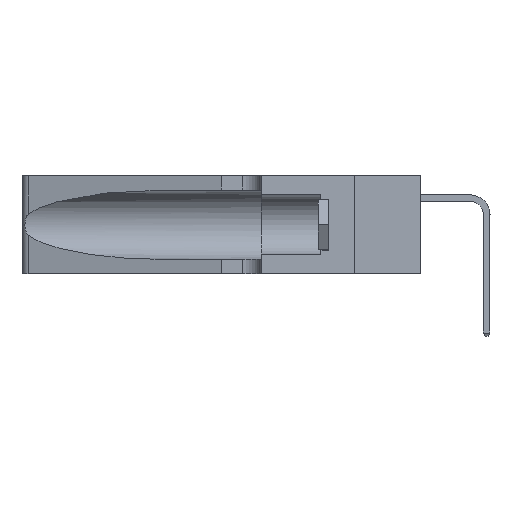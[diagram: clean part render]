
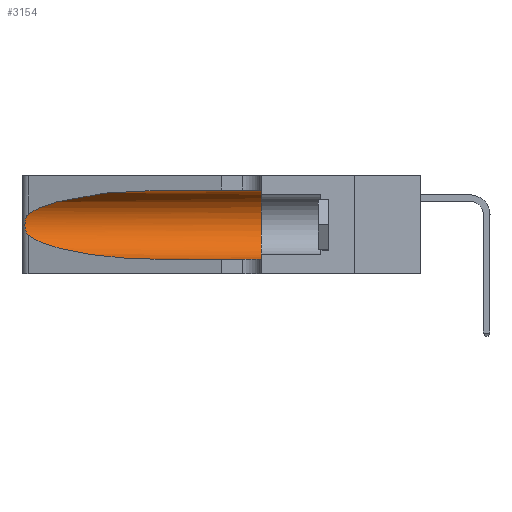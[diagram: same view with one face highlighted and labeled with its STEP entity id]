
A CAD part, left-side view. The second image highlights one B-rep face of the part: STEP entity #3154.
In plain terms, the highlighted cylindrical face has radius 3.308 mm (diameter 6.617 mm), a partial arc.
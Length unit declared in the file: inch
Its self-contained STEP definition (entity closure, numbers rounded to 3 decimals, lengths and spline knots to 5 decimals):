
#513 = CARTESIAN_POINT ( 'NONE',  ( 0.2373, 1.15595, 0.28018 ) ) ;
#948 = CARTESIAN_POINT ( 'NONE',  ( 0.25856, 1.23593, 0.16098 ) ) ;
#1229 = CARTESIAN_POINT ( 'NONE',  ( 0.1305, 1.61858, 0.31525 ) ) ;
#1253 = ORIENTED_EDGE ( 'NONE', *, *, #3445, .T. ) ;
#2383 = CARTESIAN_POINT ( 'NONE',  ( 0.25487, 1.22718, 0.22369 ) ) ;
#2447 = CARTESIAN_POINT ( 'NONE',  ( 0.25639, 1.23186, 0.15144 ) ) ;
#3079 = CYLINDRICAL_SURFACE ( 'NONE', #17905, 0.13025 ) ;
#3154 = ADVANCED_FACE ( 'NONE', ( #14807 ), #3079, .F. ) ;
#3445 = EDGE_CURVE ( 'NONE', #12646, #9688, #5342, .T. ) ;
#3483 = CARTESIAN_POINT ( 'NONE',  ( 0.1305, 1.61858, 0.185 ) ) ;
#3907 = CARTESIAN_POINT ( 'NONE',  ( 0.25487, 1.22718, 0.14631 ) ) ;
#3959 = ORIENTED_EDGE ( 'NONE', *, *, #9111, .T. ) ;
#4070 = VECTOR ( 'NONE', #13001, 39.37008 ) ;
#4878 = CARTESIAN_POINT ( 'NONE',  ( 0.1305, 0.35, 0.05475 ) ) ;
#5135 = CARTESIAN_POINT ( 'NONE',  ( 0.1305, 0.72297, 0.05475 ) ) ;
#5319 = CARTESIAN_POINT ( 'NONE',  ( 0.25639, 1.23184, 0.21858 ) ) ;
#5342 = LINE ( 'NONE', #17553, #16624 ) ;
#5837 = VERTEX_POINT ( 'NONE', #18272 ) ;
#5860 = DIRECTION ( 'NONE',  ( 0., -1., 0. ) ) ;
#6227 = ORIENTED_EDGE ( 'NONE', *, *, #8762, .F. ) ;
#6828 = CARTESIAN_POINT ( 'NONE',  ( 0.25854, 1.2359, 0.20912 ) ) ;
#7110 = DIRECTION ( 'NONE',  ( 0., 1., 0. ) ) ;
#7113 = ORIENTED_EDGE ( 'NONE', *, *, #17743, .F. ) ;
#7295 = EDGE_LOOP ( 'NONE', ( #3959, #17143, #15852, #1253, #6227, #7113 ) ) ;
#7996 = LINE ( 'NONE', #1229, #4070 ) ;
#8301 = CARTESIAN_POINT ( 'NONE',  ( 0.26075, 1.23896, 0.19203 ) ) ;
#8713 = CIRCLE ( 'NONE', #17393, 0.13025 ) ;
#8762 = EDGE_CURVE ( 'NONE', #18792, #9688, #8713, .T. ) ;
#9111 = EDGE_CURVE ( 'NONE', #12987, #5837, #9203, .T. ) ;
#9203 =( BOUNDED_CURVE ( )  B_SPLINE_CURVE ( 3, ( #15119, #15186, #513, #10826 ),
 .UNSPECIFIED., .F., .F. ) 
 B_SPLINE_CURVE_WITH_KNOTS ( ( 4, 4 ),
 ( 1.5708, 2.84003 ),
 .UNSPECIFIED. ) 
 CURVE ( )  GEOMETRIC_REPRESENTATION_ITEM ( )  RATIONAL_B_SPLINE_CURVE ( ( 1., 0.87, 0.87, 1. ) ) 
 REPRESENTATION_ITEM ( '' )  );
#9494 = CARTESIAN_POINT ( 'NONE',  ( 0.2373, 1.15595, 0.08982 ) ) ;
#9688 = VERTEX_POINT ( 'NONE', #4878 ) ;
#9752 = CARTESIAN_POINT ( 'NONE',  ( 0.26017, 1.23833, 0.17102 ) ) ;
#10818 = DIRECTION ( 'NONE',  ( 0., 0., -1. ) ) ;
#10826 = CARTESIAN_POINT ( 'NONE',  ( 0.25487, 1.22718, 0.22369 ) ) ;
#11196 = CARTESIAN_POINT ( 'NONE',  ( 0.25555, 1.22994, 0.2215 ) ) ;
#11257 = CARTESIAN_POINT ( 'NONE',  ( 0.25789, 1.23486, 0.15765 ) ) ;
#12221 = CARTESIAN_POINT ( 'NONE',  ( 0.1305, 0.72297, 0.31525 ) ) ;
#12298 = DIRECTION ( 'NONE',  ( 0., -1., 0. ) ) ;
#12478 = CARTESIAN_POINT ( 'NONE',  ( 0.25487, 1.22718, 0.14631 ) ) ;
#12646 = VERTEX_POINT ( 'NONE', #17306 ) ;
#12732 = CARTESIAN_POINT ( 'NONE',  ( 0.25555, 1.22993, 0.14849 ) ) ;
#12793 = CARTESIAN_POINT ( 'NONE',  ( 0.25487, 1.22718, 0.14631 ) ) ;
#12987 = VERTEX_POINT ( 'NONE', #12221 ) ;
#13001 = DIRECTION ( 'NONE',  ( 0., -1., 0. ) ) ;
#13111 = EDGE_CURVE ( 'NONE', #13253, #12646, #16480, .T. ) ;
#13170 = EDGE_CURVE ( 'NONE', #5837, #13253, #15645, .T. ) ;
#13253 = VERTEX_POINT ( 'NONE', #12793 ) ;
#13924 = CARTESIAN_POINT ( 'NONE',  ( 0.1305, 0.35, 0.31525 ) ) ;
#13949 = CARTESIAN_POINT ( 'NONE',  ( 0.18966, 0.96281, 0.05475 ) ) ;
#14807 = FACE_OUTER_BOUND ( 'NONE', #7295, .T. ) ;
#15119 = CARTESIAN_POINT ( 'NONE',  ( 0.1305, 0.72297, 0.31525 ) ) ;
#15186 = CARTESIAN_POINT ( 'NONE',  ( 0.18966, 0.96281, 0.31525 ) ) ;
#15618 = CARTESIAN_POINT ( 'NONE',  ( 0.25787, 1.23484, 0.2124 ) ) ;
#15645 = B_SPLINE_CURVE_WITH_KNOTS ( 'NONE', 3,
 ( #2383, #11196, #5319, #15618, #6828, #17095, #8301, #18547, #9752, #948, #11257, #2447, #12732, #3907 ),
 .UNSPECIFIED., .F., .F.,
 ( 4, 2, 2, 2, 2, 2, 4 ),
 ( 0., 0.00027, 0.00053, 0.00107, 0.0016, 0.00187, 0.00214 ),
 .UNSPECIFIED. ) ;
#15852 = ORIENTED_EDGE ( 'NONE', *, *, #13111, .T. ) ;
#15911 = CARTESIAN_POINT ( 'NONE',  ( 0.1305, 0.35, 0.185 ) ) ;
#16480 =( BOUNDED_CURVE ( )  B_SPLINE_CURVE ( 3, ( #12478, #9494, #13949, #5135 ),
 .UNSPECIFIED., .F., .F. ) 
 B_SPLINE_CURVE_WITH_KNOTS ( ( 4, 4 ),
 ( 3.44316, 4.71239 ),
 .UNSPECIFIED. ) 
 CURVE ( )  GEOMETRIC_REPRESENTATION_ITEM ( )  RATIONAL_B_SPLINE_CURVE ( ( 1., 0.87, 0.87, 1. ) ) 
 REPRESENTATION_ITEM ( '' )  );
#16624 = VECTOR ( 'NONE', #5860, 39.37008 ) ;
#17095 = CARTESIAN_POINT ( 'NONE',  ( 0.26018, 1.23835, 0.19895 ) ) ;
#17143 = ORIENTED_EDGE ( 'NONE', *, *, #13170, .T. ) ;
#17306 = CARTESIAN_POINT ( 'NONE',  ( 0.1305, 0.72297, 0.05475 ) ) ;
#17387 = DIRECTION ( 'NONE',  ( 0., 0., 1. ) ) ;
#17393 = AXIS2_PLACEMENT_3D ( 'NONE', #15911, #7110, #17387 ) ;
#17553 = CARTESIAN_POINT ( 'NONE',  ( 0.1305, 1.61858, 0.05475 ) ) ;
#17743 = EDGE_CURVE ( 'NONE', #12987, #18792, #7996, .T. ) ;
#17905 = AXIS2_PLACEMENT_3D ( 'NONE', #3483, #12298, #10818 ) ;
#18272 = CARTESIAN_POINT ( 'NONE',  ( 0.25487, 1.22718, 0.22369 ) ) ;
#18547 = CARTESIAN_POINT ( 'NONE',  ( 0.26075, 1.23896, 0.178 ) ) ;
#18792 = VERTEX_POINT ( 'NONE', #13924 ) ;
